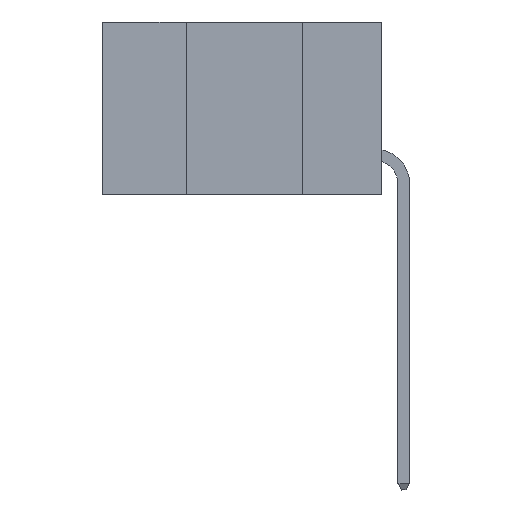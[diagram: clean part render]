
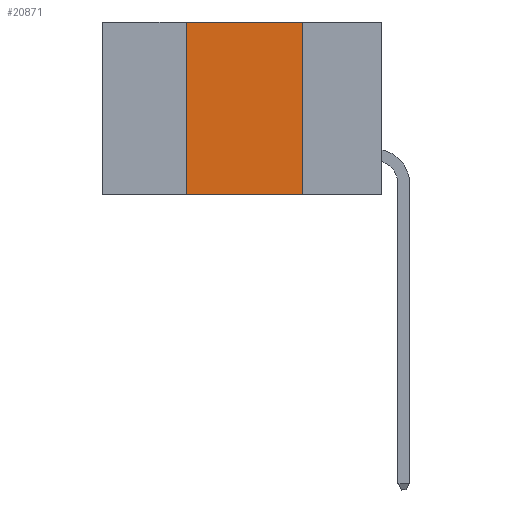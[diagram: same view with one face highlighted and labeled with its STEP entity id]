
A CAD part, left-side view. The second image highlights one B-rep face of the part: STEP entity #20871.
In plain terms, the highlighted planar face has unit normal (-1, 0, 0).
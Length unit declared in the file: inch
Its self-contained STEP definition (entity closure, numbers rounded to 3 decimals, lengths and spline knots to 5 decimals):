
#805 = VECTOR ( 'NONE', #16874, 39.37008 ) ;
#976 = DIRECTION ( 'NONE',  ( 0., 0., 1. ) ) ;
#1596 = EDGE_CURVE ( 'NONE', #11447, #15030, #11993, .T. ) ;
#2658 = CARTESIAN_POINT ( 'NONE',  ( 0., 0.17, 0. ) ) ;
#3384 = LINE ( 'NONE', #17736, #32814 ) ;
#4300 = DIRECTION ( 'NONE',  ( 0., -1., 0. ) ) ;
#10817 = DIRECTION ( 'NONE',  ( 1., 0., 0. ) ) ;
#11254 = PLANE ( 'NONE',  #34720 ) ;
#11447 = VERTEX_POINT ( 'NONE', #22843 ) ;
#11993 = LINE ( 'NONE', #37646, #805 ) ;
#12175 = ORIENTED_EDGE ( 'NONE', *, *, #16573, .F. ) ;
#12180 = EDGE_CURVE ( 'NONE', #11447, #21497, #16510, .T. ) ;
#12506 = LINE ( 'NONE', #2658, #40210 ) ;
#13838 = VECTOR ( 'NONE', #976, 39.37008 ) ;
#14274 = DIRECTION ( 'NONE',  ( 0., 0., -1. ) ) ;
#14577 = CARTESIAN_POINT ( 'NONE',  ( 0., 0.6, 0. ) ) ;
#15030 = VERTEX_POINT ( 'NONE', #43124 ) ;
#16510 = LINE ( 'NONE', #21253, #13838 ) ;
#16573 = EDGE_CURVE ( 'NONE', #26710, #15030, #12506, .T. ) ;
#16874 = DIRECTION ( 'NONE',  ( 0., -1., 0. ) ) ;
#17536 = FACE_OUTER_BOUND ( 'NONE', #31652, .T. ) ;
#17736 = CARTESIAN_POINT ( 'NONE',  ( 0., 0.6, 0. ) ) ;
#18378 = ORIENTED_EDGE ( 'NONE', *, *, #1596, .T. ) ;
#19081 = CARTESIAN_POINT ( 'NONE',  ( 0., 0.17, 0. ) ) ;
#20871 = ADVANCED_FACE ( 'NONE', ( #17536 ), #11254, .F. ) ;
#21253 = CARTESIAN_POINT ( 'NONE',  ( 0., 0.42, 0. ) ) ;
#21497 = VERTEX_POINT ( 'NONE', #37975 ) ;
#22843 = CARTESIAN_POINT ( 'NONE',  ( 0., 0.42, -0.37 ) ) ;
#23422 = DIRECTION ( 'NONE',  ( 0., 0., -1. ) ) ;
#25849 = ORIENTED_EDGE ( 'NONE', *, *, #12180, .F. ) ;
#26710 = VERTEX_POINT ( 'NONE', #19081 ) ;
#31652 = EDGE_LOOP ( 'NONE', ( #12175, #42317, #25849, #18378 ) ) ;
#32814 = VECTOR ( 'NONE', #4300, 39.37008 ) ;
#33371 = EDGE_CURVE ( 'NONE', #21497, #26710, #3384, .T. ) ;
#34720 = AXIS2_PLACEMENT_3D ( 'NONE', #14577, #10817, #14274 ) ;
#37646 = CARTESIAN_POINT ( 'NONE',  ( 0., 0.6, -0.37 ) ) ;
#37975 = CARTESIAN_POINT ( 'NONE',  ( 0., 0.42, 0. ) ) ;
#40210 = VECTOR ( 'NONE', #23422, 39.37008 ) ;
#42317 = ORIENTED_EDGE ( 'NONE', *, *, #33371, .F. ) ;
#43124 = CARTESIAN_POINT ( 'NONE',  ( 0., 0.17, -0.37 ) ) ;
